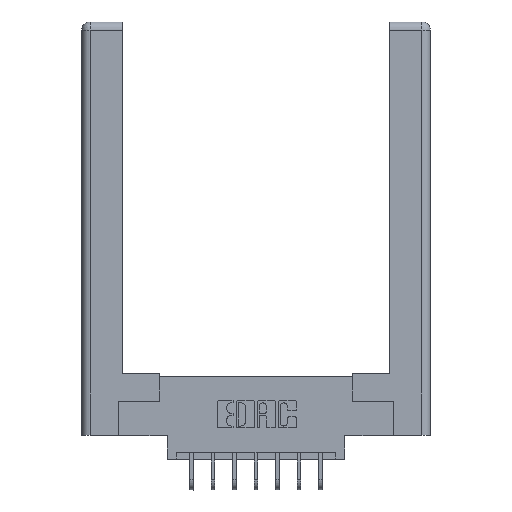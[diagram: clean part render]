
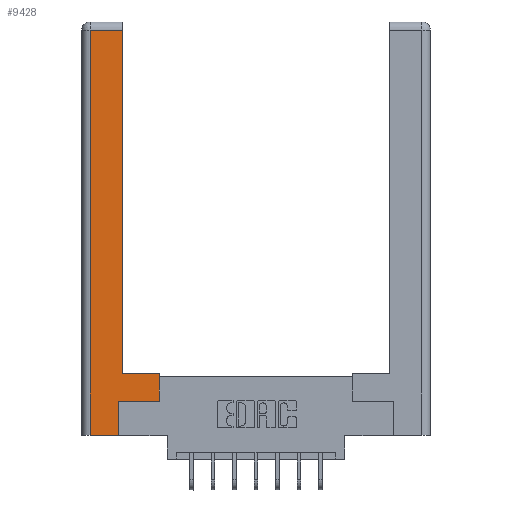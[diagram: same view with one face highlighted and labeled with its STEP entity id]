
A CAD part, top view. The second image highlights one B-rep face of the part: STEP entity #9428.
In plain terms, the highlighted planar face has unit normal (0, 0, 1).
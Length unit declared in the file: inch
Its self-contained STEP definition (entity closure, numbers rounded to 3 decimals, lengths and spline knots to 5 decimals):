
#890 = LINE ( 'NONE', #1171, #4685 ) ;
#1169 = DIRECTION ( 'NONE',  ( 1., 0., 0. ) ) ;
#1171 = CARTESIAN_POINT ( 'NONE',  ( 0.265, 0.245, 0. ) ) ;
#1217 = VERTEX_POINT ( 'NONE', #13046 ) ;
#1237 = VECTOR ( 'NONE', #10076, 39.37008 ) ;
#1344 = CARTESIAN_POINT ( 'NONE',  ( 0.0615, 2.94, 0. ) ) ;
#1575 = LINE ( 'NONE', #8923, #1237 ) ;
#1586 = VERTEX_POINT ( 'NONE', #13328 ) ;
#2024 = EDGE_CURVE ( 'NONE', #7040, #7561, #3759, .T. ) ;
#3027 = CARTESIAN_POINT ( 'NONE',  ( 0.565, 0.245, 0. ) ) ;
#3547 = PLANE ( 'NONE',  #13077 ) ;
#3564 = EDGE_CURVE ( 'NONE', #13023, #7040, #1575, .T. ) ;
#3759 = LINE ( 'NONE', #7994, #4973 ) ;
#4414 = ORIENTED_EDGE ( 'NONE', *, *, #2024, .T. ) ;
#4583 = VERTEX_POINT ( 'NONE', #3027 ) ;
#4685 = VECTOR ( 'NONE', #13672, 39.37008 ) ;
#4973 = VECTOR ( 'NONE', #11688, 39.37008 ) ;
#5257 = EDGE_CURVE ( 'NONE', #1217, #4583, #9043, .T. ) ;
#5358 = LINE ( 'NONE', #7848, #14004 ) ;
#6033 = EDGE_CURVE ( 'NONE', #1586, #12654, #10393, .T. ) ;
#6557 = ORIENTED_EDGE ( 'NONE', *, *, #6033, .T. ) ;
#6900 = DIRECTION ( 'NONE',  ( 0., 0., -1. ) ) ;
#6981 = EDGE_LOOP ( 'NONE', ( #13942, #10666, #4414, #12208, #14473, #14524, #9625, #6557 ) ) ;
#7040 = VERTEX_POINT ( 'NONE', #1344 ) ;
#7236 = DIRECTION ( 'NONE',  ( -1., 0., 0. ) ) ;
#7275 = CARTESIAN_POINT ( 'NONE',  ( 0.0615, 0., 0. ) ) ;
#7312 = DIRECTION ( 'NONE',  ( 0., 1., 0. ) ) ;
#7561 = VERTEX_POINT ( 'NONE', #7275 ) ;
#7848 = CARTESIAN_POINT ( 'NONE',  ( 0.265, 0., 0. ) ) ;
#7972 = DIRECTION ( 'NONE',  ( -1., 0., 0. ) ) ;
#7994 = CARTESIAN_POINT ( 'NONE',  ( 0.0615, 0., 0. ) ) ;
#8084 = CARTESIAN_POINT ( 'NONE',  ( 0., 0., 0. ) ) ;
#8923 = CARTESIAN_POINT ( 'NONE',  ( 0.0615, 2.94, 0. ) ) ;
#9043 = LINE ( 'NONE', #12880, #11363 ) ;
#9428 = ADVANCED_FACE ( 'NONE', ( #9460 ), #3547, .F. ) ;
#9460 = FACE_OUTER_BOUND ( 'NONE', #6981, .T. ) ;
#9558 = CARTESIAN_POINT ( 'NONE',  ( 0.295, 0.45, 0. ) ) ;
#9615 = VECTOR ( 'NONE', #7312, 39.37008 ) ;
#9625 = ORIENTED_EDGE ( 'NONE', *, *, #10154, .T. ) ;
#10076 = DIRECTION ( 'NONE',  ( -1., 0., 0. ) ) ;
#10154 = EDGE_CURVE ( 'NONE', #4583, #1586, #10509, .T. ) ;
#10393 = LINE ( 'NONE', #11537, #13758 ) ;
#10509 = LINE ( 'NONE', #12711, #9615 ) ;
#10553 = CARTESIAN_POINT ( 'NONE',  ( 0.295, 2.94, 0. ) ) ;
#10666 = ORIENTED_EDGE ( 'NONE', *, *, #3564, .T. ) ;
#10707 = DIRECTION ( 'NONE',  ( 1., 0., 0. ) ) ;
#11170 = EDGE_CURVE ( 'NONE', #12654, #13023, #13144, .T. ) ;
#11262 = EDGE_CURVE ( 'NONE', #7561, #14442, #5358, .T. ) ;
#11363 = VECTOR ( 'NONE', #10707, 39.37008 ) ;
#11537 = CARTESIAN_POINT ( 'NONE',  ( 0.295, 0.45, 0. ) ) ;
#11688 = DIRECTION ( 'NONE',  ( 0., -1., 0. ) ) ;
#11817 = CARTESIAN_POINT ( 'NONE',  ( 0.295, 3., 0. ) ) ;
#12208 = ORIENTED_EDGE ( 'NONE', *, *, #11262, .T. ) ;
#12305 = CARTESIAN_POINT ( 'NONE',  ( 0.265, 0., 0. ) ) ;
#12654 = VERTEX_POINT ( 'NONE', #9558 ) ;
#12711 = CARTESIAN_POINT ( 'NONE',  ( 0.565, 0.45, 0. ) ) ;
#12779 = VECTOR ( 'NONE', #12920, 39.37008 ) ;
#12852 = EDGE_CURVE ( 'NONE', #14442, #1217, #890, .T. ) ;
#12880 = CARTESIAN_POINT ( 'NONE',  ( 0.565, 0.245, 0. ) ) ;
#12920 = DIRECTION ( 'NONE',  ( 0., 1., 0. ) ) ;
#13023 = VERTEX_POINT ( 'NONE', #10553 ) ;
#13046 = CARTESIAN_POINT ( 'NONE',  ( 0.265, 0.245, 0. ) ) ;
#13077 = AXIS2_PLACEMENT_3D ( 'NONE', #8084, #6900, #7972 ) ;
#13144 = LINE ( 'NONE', #11817, #12779 ) ;
#13328 = CARTESIAN_POINT ( 'NONE',  ( 0.565, 0.45, 0. ) ) ;
#13672 = DIRECTION ( 'NONE',  ( 0., 1., 0. ) ) ;
#13758 = VECTOR ( 'NONE', #7236, 39.37008 ) ;
#13942 = ORIENTED_EDGE ( 'NONE', *, *, #11170, .T. ) ;
#14004 = VECTOR ( 'NONE', #1169, 39.37008 ) ;
#14442 = VERTEX_POINT ( 'NONE', #12305 ) ;
#14473 = ORIENTED_EDGE ( 'NONE', *, *, #12852, .T. ) ;
#14524 = ORIENTED_EDGE ( 'NONE', *, *, #5257, .T. ) ;
